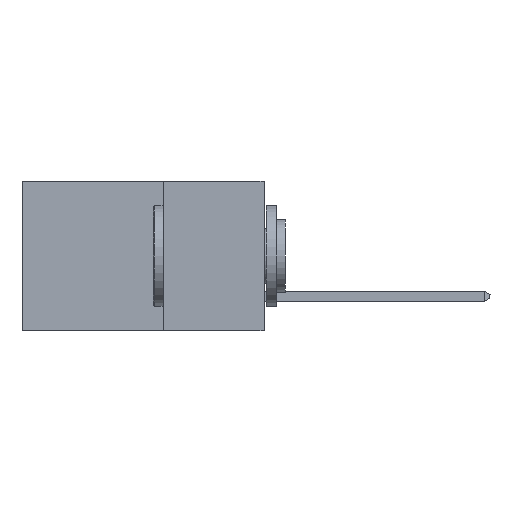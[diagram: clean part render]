
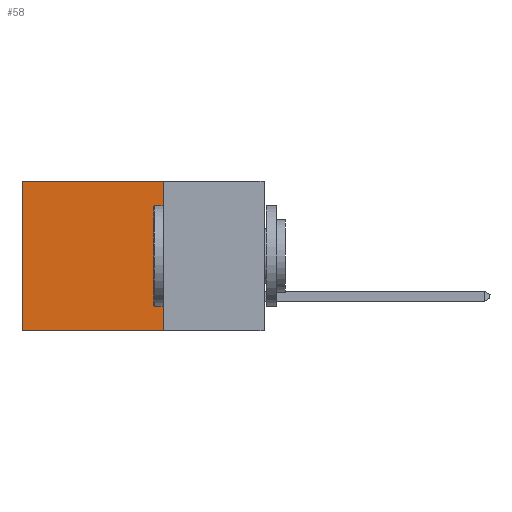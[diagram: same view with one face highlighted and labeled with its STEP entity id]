
A CAD part, left-side view. The second image highlights one B-rep face of the part: STEP entity #58.
In plain terms, the highlighted planar face has unit normal (-1, 0, 0).
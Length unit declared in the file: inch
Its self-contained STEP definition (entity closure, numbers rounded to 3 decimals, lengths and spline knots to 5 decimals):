
#58 = ADVANCED_FACE ( 'NONE', ( #4974 ), #7932, .F. ) ;
#239 = DIRECTION ( 'NONE',  ( 1., 0., 0. ) ) ;
#385 = EDGE_CURVE ( 'NONE', #731, #5784, #8073, .T. ) ;
#731 = VERTEX_POINT ( 'NONE', #910 ) ;
#737 = ORIENTED_EDGE ( 'NONE', *, *, #5162, .F. ) ;
#900 = LINE ( 'NONE', #2042, #3669 ) ;
#910 = CARTESIAN_POINT ( 'NONE',  ( 0.298, 0.25, 0. ) ) ;
#1858 = LINE ( 'NONE', #6006, #9126 ) ;
#1938 = DIRECTION ( 'NONE',  ( 0., 0., -1. ) ) ;
#1942 = AXIS2_PLACEMENT_3D ( 'NONE', #5690, #239, #2640 ) ;
#2042 = CARTESIAN_POINT ( 'NONE',  ( 0.298, 0.6, 0. ) ) ;
#2640 = DIRECTION ( 'NONE',  ( 0., 0., -1. ) ) ;
#2913 = VERTEX_POINT ( 'NONE', #3509 ) ;
#3456 = CARTESIAN_POINT ( 'NONE',  ( 0.298, 0.25, 0. ) ) ;
#3509 = CARTESIAN_POINT ( 'NONE',  ( 0.298, 0.6, -0.37 ) ) ;
#3557 = DIRECTION ( 'NONE',  ( 0., 0., -1. ) ) ;
#3669 = VECTOR ( 'NONE', #3557, 39.37008 ) ;
#3938 = CARTESIAN_POINT ( 'NONE',  ( 0.298, 0.25, 0. ) ) ;
#4974 = FACE_OUTER_BOUND ( 'NONE', #5146, .T. ) ;
#5132 = CARTESIAN_POINT ( 'NONE',  ( 0.298, 0.25, -0.37 ) ) ;
#5146 = EDGE_LOOP ( 'NONE', ( #7044, #737, #6000, #8917 ) ) ;
#5162 = EDGE_CURVE ( 'NONE', #6993, #2913, #1858, .T. ) ;
#5690 = CARTESIAN_POINT ( 'NONE',  ( 0.298, 0.25, 0. ) ) ;
#5784 = VERTEX_POINT ( 'NONE', #9229 ) ;
#5968 = DIRECTION ( 'NONE',  ( 0., 1., 0. ) ) ;
#6000 = ORIENTED_EDGE ( 'NONE', *, *, #6113, .F. ) ;
#6006 = CARTESIAN_POINT ( 'NONE',  ( 0.298, 0.25, -0.37 ) ) ;
#6082 = EDGE_CURVE ( 'NONE', #5784, #2913, #900, .T. ) ;
#6113 = EDGE_CURVE ( 'NONE', #731, #6993, #7378, .T. ) ;
#6120 = DIRECTION ( 'NONE',  ( 0., 1., 0. ) ) ;
#6993 = VERTEX_POINT ( 'NONE', #5132 ) ;
#7044 = ORIENTED_EDGE ( 'NONE', *, *, #6082, .T. ) ;
#7378 = LINE ( 'NONE', #3456, #9453 ) ;
#7481 = VECTOR ( 'NONE', #6120, 39.37008 ) ;
#7932 = PLANE ( 'NONE',  #1942 ) ;
#8073 = LINE ( 'NONE', #3938, #7481 ) ;
#8917 = ORIENTED_EDGE ( 'NONE', *, *, #385, .T. ) ;
#9126 = VECTOR ( 'NONE', #5968, 39.37008 ) ;
#9229 = CARTESIAN_POINT ( 'NONE',  ( 0.298, 0.6, 0. ) ) ;
#9453 = VECTOR ( 'NONE', #1938, 39.37008 ) ;
